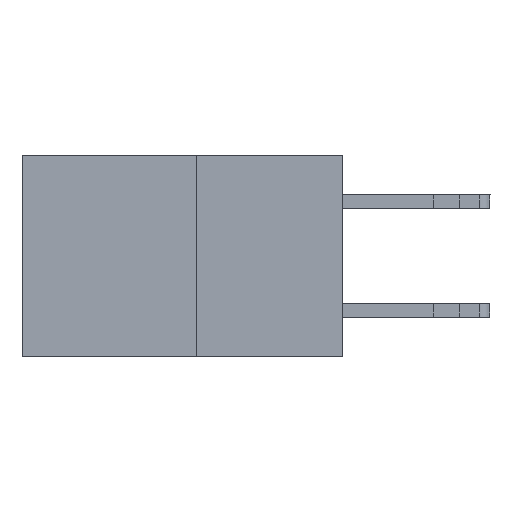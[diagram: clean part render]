
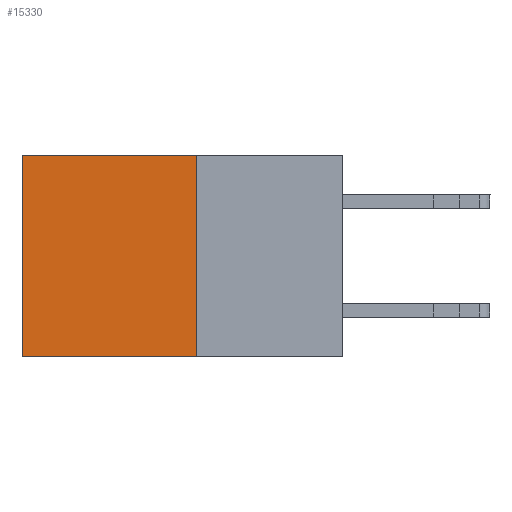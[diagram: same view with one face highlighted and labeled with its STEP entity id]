
A CAD part, left-side view. The second image highlights one B-rep face of the part: STEP entity #15330.
In plain terms, the highlighted planar face has unit normal (-1, 0, 0).
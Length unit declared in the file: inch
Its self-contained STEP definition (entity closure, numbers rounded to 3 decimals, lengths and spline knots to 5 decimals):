
#1147 = DIRECTION ( 'NONE',  ( 0., 1., 0. ) ) ;
#1565 = CARTESIAN_POINT ( 'NONE',  ( 0.277, 0.27, -0.37 ) ) ;
#1671 = VECTOR ( 'NONE', #5245, 39.37008 ) ;
#1713 = DIRECTION ( 'NONE',  ( 1., 0., 0. ) ) ;
#1880 = CARTESIAN_POINT ( 'NONE',  ( 0.277, 0.27, -0.37 ) ) ;
#1969 = ORIENTED_EDGE ( 'NONE', *, *, #14244, .F. ) ;
#2472 = EDGE_LOOP ( 'NONE', ( #7617, #1969, #9826, #9414 ) ) ;
#2802 = VECTOR ( 'NONE', #1147, 39.37008 ) ;
#2809 = DIRECTION ( 'NONE',  ( 0., 0., -1. ) ) ;
#3987 = CARTESIAN_POINT ( 'NONE',  ( 0.277, 0.59, -0.37 ) ) ;
#4506 = CARTESIAN_POINT ( 'NONE',  ( 0.277, 0.27, 0. ) ) ;
#4540 = LINE ( 'NONE', #1880, #9712 ) ;
#4580 = AXIS2_PLACEMENT_3D ( 'NONE', #10113, #1713, #11284 ) ;
#5245 = DIRECTION ( 'NONE',  ( 0., 1., 0. ) ) ;
#5927 = VERTEX_POINT ( 'NONE', #1565 ) ;
#6063 = VERTEX_POINT ( 'NONE', #15383 ) ;
#6450 = CARTESIAN_POINT ( 'NONE',  ( 0.277, 0.59, 0. ) ) ;
#6453 = VERTEX_POINT ( 'NONE', #4506 ) ;
#7617 = ORIENTED_EDGE ( 'NONE', *, *, #8730, .T. ) ;
#8291 = CARTESIAN_POINT ( 'NONE',  ( 0.277, 0.27, -0.37 ) ) ;
#8730 = EDGE_CURVE ( 'NONE', #10147, #6063, #12384, .T. ) ;
#8749 = EDGE_CURVE ( 'NONE', #6453, #10147, #12469, .T. ) ;
#9333 = DIRECTION ( 'NONE',  ( 0., 0., -1. ) ) ;
#9414 = ORIENTED_EDGE ( 'NONE', *, *, #8749, .T. ) ;
#9712 = VECTOR ( 'NONE', #9333, 39.37008 ) ;
#9826 = ORIENTED_EDGE ( 'NONE', *, *, #11350, .F. ) ;
#9960 = CARTESIAN_POINT ( 'NONE',  ( 0.277, 0.27, 0. ) ) ;
#10113 = CARTESIAN_POINT ( 'NONE',  ( 0.277, 0.27, -0.37 ) ) ;
#10147 = VERTEX_POINT ( 'NONE', #6450 ) ;
#11284 = DIRECTION ( 'NONE',  ( 0., 0., -1. ) ) ;
#11350 = EDGE_CURVE ( 'NONE', #6453, #5927, #4540, .T. ) ;
#12159 = PLANE ( 'NONE',  #4580 ) ;
#12384 = LINE ( 'NONE', #3987, #15235 ) ;
#12469 = LINE ( 'NONE', #9960, #1671 ) ;
#14244 = EDGE_CURVE ( 'NONE', #5927, #6063, #15455, .T. ) ;
#14834 = FACE_OUTER_BOUND ( 'NONE', #2472, .T. ) ;
#15235 = VECTOR ( 'NONE', #2809, 39.37008 ) ;
#15330 = ADVANCED_FACE ( 'NONE', ( #14834 ), #12159, .F. ) ;
#15383 = CARTESIAN_POINT ( 'NONE',  ( 0.277, 0.59, -0.37 ) ) ;
#15455 = LINE ( 'NONE', #8291, #2802 ) ;
